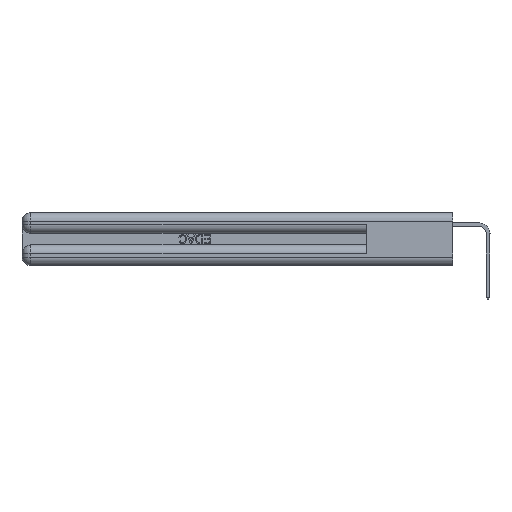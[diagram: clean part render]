
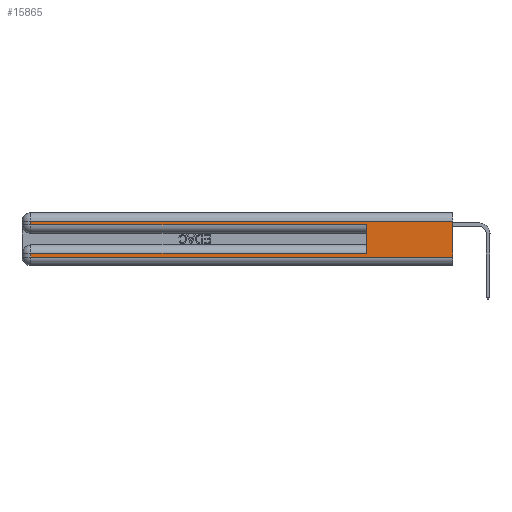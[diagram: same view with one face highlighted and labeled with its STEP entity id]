
A CAD part, left-side view. The second image highlights one B-rep face of the part: STEP entity #15865.
In plain terms, the highlighted planar face has unit normal (-1, 0, 0).
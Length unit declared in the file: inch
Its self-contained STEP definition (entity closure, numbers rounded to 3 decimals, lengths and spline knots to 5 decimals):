
#129 = LINE ( 'NONE', #37747, #16811 ) ;
#928 = CARTESIAN_POINT ( 'NONE',  ( 0., 0., 0.06 ) ) ;
#1011 = VERTEX_POINT ( 'NONE', #7490 ) ;
#1339 = CARTESIAN_POINT ( 'NONE',  ( 0., 2.94, 0.37 ) ) ;
#1459 = ORIENTED_EDGE ( 'NONE', *, *, #2184, .F. ) ;
#1785 = CARTESIAN_POINT ( 'NONE',  ( 0., 2.94, 0.31 ) ) ;
#2184 = EDGE_CURVE ( 'NONE', #37641, #4139, #20445, .T. ) ;
#2964 = VECTOR ( 'NONE', #3894, 39.37008 ) ;
#3318 = EDGE_CURVE ( 'NONE', #1011, #5338, #16718, .T. ) ;
#3786 = ORIENTED_EDGE ( 'NONE', *, *, #3318, .F. ) ;
#3894 = DIRECTION ( 'NONE',  ( 0., -1., 0. ) ) ;
#4067 = LINE ( 'NONE', #29925, #28474 ) ;
#4139 = VERTEX_POINT ( 'NONE', #928 ) ;
#4288 = CARTESIAN_POINT ( 'NONE',  ( 0., 0., 0.37 ) ) ;
#4293 = CARTESIAN_POINT ( 'NONE',  ( 0., 0., 0.085 ) ) ;
#4912 = ORIENTED_EDGE ( 'NONE', *, *, #36605, .T. ) ;
#5338 = VERTEX_POINT ( 'NONE', #34172 ) ;
#5407 = EDGE_CURVE ( 'NONE', #31846, #21267, #129, .T. ) ;
#5466 = CARTESIAN_POINT ( 'NONE',  ( 0., 0., 0.31 ) ) ;
#6395 = LINE ( 'NONE', #1339, #31834 ) ;
#6863 = CARTESIAN_POINT ( 'NONE',  ( 0., 0.6, 0.145 ) ) ;
#7490 = CARTESIAN_POINT ( 'NONE',  ( 0., 0.6, 0.085 ) ) ;
#11013 = CARTESIAN_POINT ( 'NONE',  ( 0., 0., 0.37 ) ) ;
#12681 = VECTOR ( 'NONE', #21010, 39.37008 ) ;
#13063 = LINE ( 'NONE', #33307, #30704 ) ;
#13379 = DIRECTION ( 'NONE',  ( 0., 1., 0. ) ) ;
#14331 = DIRECTION ( 'NONE',  ( 0., 0., -1. ) ) ;
#14339 = DIRECTION ( 'NONE',  ( 0., 1., 0. ) ) ;
#15865 = ADVANCED_FACE ( 'NONE', ( #29818 ), #30875, .F. ) ;
#16718 = LINE ( 'NONE', #6863, #25524 ) ;
#16811 = VECTOR ( 'NONE', #34581, 39.37008 ) ;
#17111 = CARTESIAN_POINT ( 'NONE',  ( 0., 0., 0.285 ) ) ;
#18835 = ORIENTED_EDGE ( 'NONE', *, *, #22489, .T. ) ;
#18924 = ORIENTED_EDGE ( 'NONE', *, *, #21910, .T. ) ;
#20445 = LINE ( 'NONE', #11013, #12681 ) ;
#20746 = ORIENTED_EDGE ( 'NONE', *, *, #32813, .T. ) ;
#21010 = DIRECTION ( 'NONE',  ( 0., 0., -1. ) ) ;
#21267 = VERTEX_POINT ( 'NONE', #41355 ) ;
#21910 = EDGE_CURVE ( 'NONE', #35615, #28071, #6395, .T. ) ;
#22489 = EDGE_CURVE ( 'NONE', #21267, #5338, #29488, .T. ) ;
#23169 = EDGE_CURVE ( 'NONE', #1011, #35615, #29942, .T. ) ;
#23325 = EDGE_LOOP ( 'NONE', ( #1459, #20746, #31166, #18835, #3786, #40681, #18924, #4912 ) ) ;
#25524 = VECTOR ( 'NONE', #26718, 39.37008 ) ;
#26267 = CARTESIAN_POINT ( 'NONE',  ( 0., 2.94, 0.06 ) ) ;
#26718 = DIRECTION ( 'NONE',  ( 0., 0., 1. ) ) ;
#28071 = VERTEX_POINT ( 'NONE', #26267 ) ;
#28474 = VECTOR ( 'NONE', #13379, 39.37008 ) ;
#29488 = LINE ( 'NONE', #17111, #2964 ) ;
#29818 = FACE_OUTER_BOUND ( 'NONE', #23325, .T. ) ;
#29925 = CARTESIAN_POINT ( 'NONE',  ( 0., 0., 0.31 ) ) ;
#29942 = LINE ( 'NONE', #4293, #37686 ) ;
#30704 = VECTOR ( 'NONE', #36643, 39.37008 ) ;
#30875 = PLANE ( 'NONE',  #41993 ) ;
#31148 = DIRECTION ( 'NONE',  ( 0., 0., -1. ) ) ;
#31166 = ORIENTED_EDGE ( 'NONE', *, *, #5407, .T. ) ;
#31834 = VECTOR ( 'NONE', #31148, 39.37008 ) ;
#31846 = VERTEX_POINT ( 'NONE', #1785 ) ;
#32813 = EDGE_CURVE ( 'NONE', #37641, #31846, #4067, .T. ) ;
#33307 = CARTESIAN_POINT ( 'NONE',  ( 0., 0., 0.06 ) ) ;
#34172 = CARTESIAN_POINT ( 'NONE',  ( 0., 0.6, 0.285 ) ) ;
#34214 = DIRECTION ( 'NONE',  ( 1., 0., 0. ) ) ;
#34581 = DIRECTION ( 'NONE',  ( 0., 0., -1. ) ) ;
#35615 = VERTEX_POINT ( 'NONE', #42307 ) ;
#36605 = EDGE_CURVE ( 'NONE', #28071, #4139, #13063, .T. ) ;
#36643 = DIRECTION ( 'NONE',  ( 0., -1., 0. ) ) ;
#37641 = VERTEX_POINT ( 'NONE', #5466 ) ;
#37686 = VECTOR ( 'NONE', #14339, 39.37008 ) ;
#37747 = CARTESIAN_POINT ( 'NONE',  ( 0., 2.94, 0.37 ) ) ;
#40681 = ORIENTED_EDGE ( 'NONE', *, *, #23169, .T. ) ;
#41355 = CARTESIAN_POINT ( 'NONE',  ( 0., 2.94, 0.285 ) ) ;
#41993 = AXIS2_PLACEMENT_3D ( 'NONE', #4288, #34214, #14331 ) ;
#42307 = CARTESIAN_POINT ( 'NONE',  ( 0., 2.94, 0.085 ) ) ;
